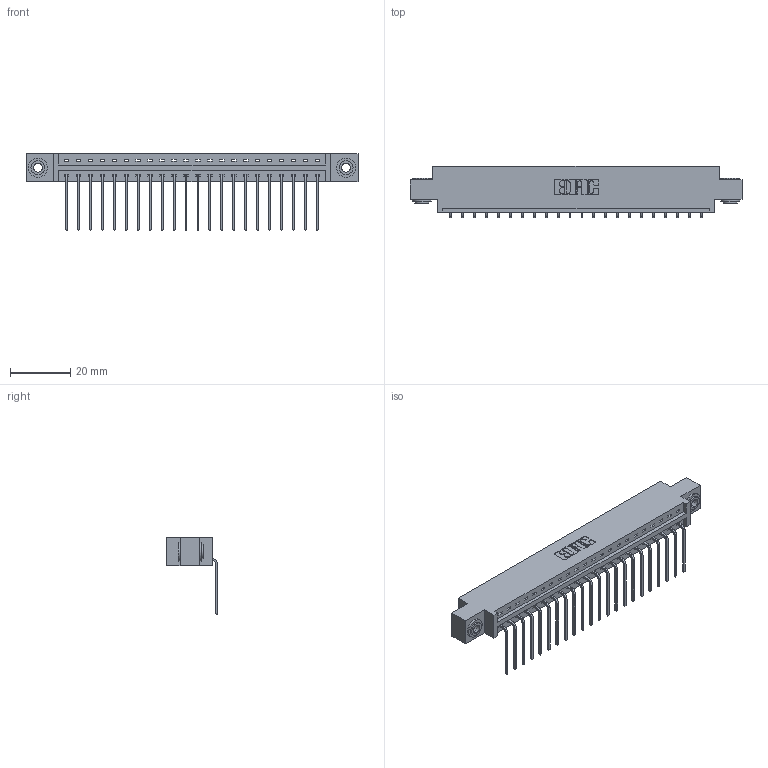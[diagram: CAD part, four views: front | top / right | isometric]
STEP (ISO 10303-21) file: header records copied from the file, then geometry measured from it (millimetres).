
FILE_DESCRIPTION (( 'STEP AP203' ), '1' );
FILE_NAME ('337-022-559-603.STEP', '2019-09-30T14:07:26', ( '' ), ( '' ), 'SwSTEP 2.0', 'SolidWorks 2016', '' );
FILE_SCHEMA (( 'CONFIG_CONTROL_DESIGN' ));
Length unit declared in the file: inch
Products named in the file (4): 345-292-001_558 559 Tail - 1; 337 Part_0.170 Offset - 0.156 Dia-TH; 337-022-559-603; 345-250-002_345-250-002-102
Assembly tree (25 placements, depth 2):
  337-022-559-603
    337 Part_0.170 Offset - 0.156 Dia-TH
    345-292-001_558 559 Tail - 1  x22
    345-250-002_345-250-002-102  x2
Bounding box: 110.19 x 17.09 x 25.53 mm (x, y, z)
Volume: 11176.8 mm3; surface area: 12218 mm2
Topology: 25 solids, 25 shells, 1564 faces, 4667 edges, 3078 vertices
Faces by surface type: plane 1140, cylinder 416, cone 8
Entity records: 19806 total; most frequent: CARTESIAN_POINT 3427, ORIENTED_EDGE 3378, DIRECTION 2959, EDGE_CURVE 1689, VECTOR 1537, LINE 1537, VERTEX_POINT 1122, AXIS2_PLACEMENT_3D 711
